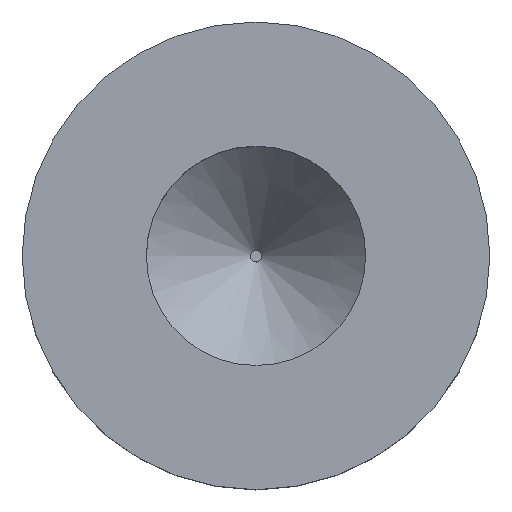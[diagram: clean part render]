
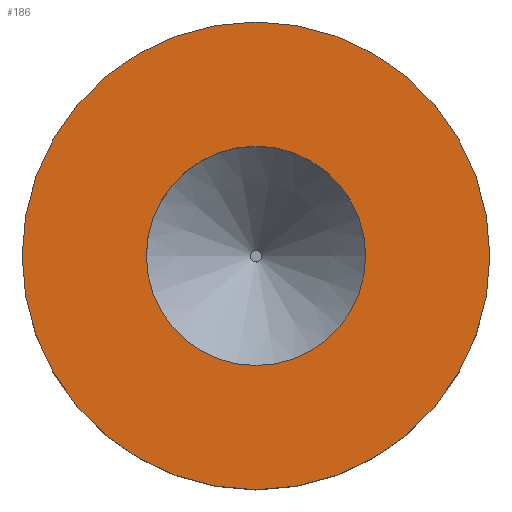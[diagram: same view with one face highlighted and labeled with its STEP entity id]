
A CAD part, top view. The second image highlights one B-rep face of the part: STEP entity #186.
In plain terms, the highlighted planar face has unit normal (0, 0, 1).
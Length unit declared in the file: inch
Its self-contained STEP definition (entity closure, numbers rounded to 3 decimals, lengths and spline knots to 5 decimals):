
#10 = DIRECTION ( 'NONE',  ( 0., 0., 1. ) ) ;
#11 = CARTESIAN_POINT ( 'NONE',  ( 0., 0., 0.25 ) ) ;
#14 = CARTESIAN_POINT ( 'NONE',  ( 0.225, 0., 0.25 ) ) ;
#19 = DIRECTION ( 'NONE',  ( 1., 0., 0. ) ) ;
#38 = AXIS2_PLACEMENT_3D ( 'NONE', #86, #10, #54 ) ;
#54 = DIRECTION ( 'NONE',  ( 1., 0., 0. ) ) ;
#55 = EDGE_LOOP ( 'NONE', ( #182 ) ) ;
#71 = DIRECTION ( 'NONE',  ( 0., 0., 1. ) ) ;
#74 = ORIENTED_EDGE ( 'NONE', *, *, #82, .F. ) ;
#80 = AXIS2_PLACEMENT_3D ( 'NONE', #11, #71, #19 ) ;
#82 = EDGE_CURVE ( 'NONE', #120, #120, #135, .T. ) ;
#86 = CARTESIAN_POINT ( 'NONE',  ( 0., 0., 0.25 ) ) ;
#87 = AXIS2_PLACEMENT_3D ( 'NONE', #141, #112, #94 ) ;
#94 = DIRECTION ( 'NONE',  ( 1., 0., 0. ) ) ;
#111 = CARTESIAN_POINT ( 'NONE',  ( 0.1055, 0., 0.25 ) ) ;
#112 = DIRECTION ( 'NONE',  ( 0., 0., 1. ) ) ;
#114 = VERTEX_POINT ( 'NONE', #14 ) ;
#120 = VERTEX_POINT ( 'NONE', #111 ) ;
#124 = FACE_BOUND ( 'NONE', #181, .T. ) ;
#130 = FACE_OUTER_BOUND ( 'NONE', #55, .T. ) ;
#135 = CIRCLE ( 'NONE', #80, 0.1055 ) ;
#141 = CARTESIAN_POINT ( 'NONE',  ( 0., 0., 0.25 ) ) ;
#147 = CIRCLE ( 'NONE', #87, 0.225 ) ;
#157 = EDGE_CURVE ( 'NONE', #114, #114, #147, .T. ) ;
#165 = PLANE ( 'NONE',  #38 ) ;
#181 = EDGE_LOOP ( 'NONE', ( #74 ) ) ;
#182 = ORIENTED_EDGE ( 'NONE', *, *, #157, .T. ) ;
#186 = ADVANCED_FACE ( 'NONE', ( #130, #124 ), #165, .T. ) ;
